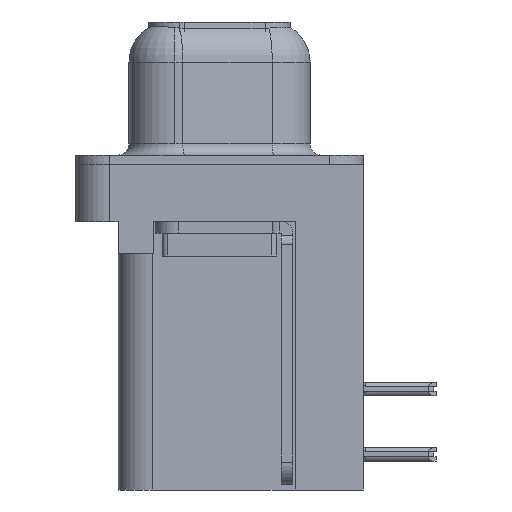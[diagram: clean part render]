
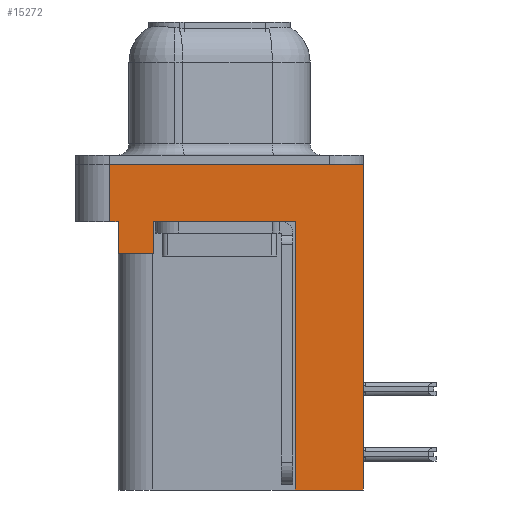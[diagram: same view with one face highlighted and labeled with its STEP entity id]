
A CAD part, left-side view. The second image highlights one B-rep face of the part: STEP entity #15272.
In plain terms, the highlighted planar face has unit normal (-1, 0, 0).
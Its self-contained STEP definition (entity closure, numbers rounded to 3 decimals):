
#4 = LINE ( 'NONE', #18601, #1381 ) ;
#1381 = VECTOR ( 'NONE', #23436, 1000. ) ;
#2305 = VERTEX_POINT ( 'NONE', #29131 ) ;
#3028 = EDGE_CURVE ( 'NONE', #26941, #27357, #26140, .T. ) ;
#3151 = EDGE_CURVE ( 'NONE', #13472, #6666, #7966, .T. ) ;
#3356 = LINE ( 'NONE', #11405, #26285 ) ;
#3766 = DIRECTION ( 'NONE',  ( 0., 0., 1. ) ) ;
#3957 = ORIENTED_EDGE ( 'NONE', *, *, #4038, .F. ) ;
#4038 = EDGE_CURVE ( 'NONE', #20231, #8632, #13422, .T. ) ;
#4247 = CARTESIAN_POINT ( 'NONE',  ( -3., 2.895, -3.9 ) ) ;
#4340 = VERTEX_POINT ( 'NONE', #17280 ) ;
#4363 = CARTESIAN_POINT ( 'NONE',  ( -3., 4.425, -3.9 ) ) ;
#4394 = EDGE_CURVE ( 'NONE', #6666, #2305, #20067, .T. ) ;
#4581 = DIRECTION ( 'NONE',  ( 0., 1., 0. ) ) ;
#4609 = CARTESIAN_POINT ( 'NONE',  ( -3., 4.425, -2.5 ) ) ;
#4730 = LINE ( 'NONE', #12021, #21700 ) ;
#4919 = VECTOR ( 'NONE', #22913, 1000. ) ;
#5632 = DIRECTION ( 'NONE',  ( 0., -1., 0. ) ) ;
#5681 = VECTOR ( 'NONE', #7447, 1000. ) ;
#5896 = CARTESIAN_POINT ( 'NONE',  ( -3., -6.275, -14.2 ) ) ;
#6021 = ORIENTED_EDGE ( 'NONE', *, *, #4394, .T. ) ;
#6219 = DIRECTION ( 'NONE',  ( 0., 1., 0. ) ) ;
#6666 = VERTEX_POINT ( 'NONE', #14466 ) ;
#7362 = DIRECTION ( 'NONE',  ( 0., 0., 1. ) ) ;
#7447 = DIRECTION ( 'NONE',  ( 0., 0., 1. ) ) ;
#7614 = PLANE ( 'NONE',  #14154 ) ;
#7671 = ORIENTED_EDGE ( 'NONE', *, *, #15102, .T. ) ;
#7966 = LINE ( 'NONE', #8420, #30158 ) ;
#8420 = CARTESIAN_POINT ( 'NONE',  ( -3., 2.895, -3.9 ) ) ;
#8632 = VERTEX_POINT ( 'NONE', #16535 ) ;
#8989 = CARTESIAN_POINT ( 'NONE',  ( -3., 4.425, -3.9 ) ) ;
#9892 = VECTOR ( 'NONE', #5632, 1000. ) ;
#10403 = VERTEX_POINT ( 'NONE', #5896 ) ;
#11405 = CARTESIAN_POINT ( 'NONE',  ( -3., -3.295, -14.2 ) ) ;
#12021 = CARTESIAN_POINT ( 'NONE',  ( -3., 4.775, -2.5 ) ) ;
#12225 = VECTOR ( 'NONE', #23926, 1000. ) ;
#12559 = CARTESIAN_POINT ( 'NONE',  ( -3., -6.275, -2.5 ) ) ;
#13422 = LINE ( 'NONE', #27539, #4919 ) ;
#13472 = VERTEX_POINT ( 'NONE', #4247 ) ;
#13940 = EDGE_CURVE ( 'NONE', #13472, #26941, #20506, .T. ) ;
#14154 = AXIS2_PLACEMENT_3D ( 'NONE', #12559, #17077, #26540 ) ;
#14466 = CARTESIAN_POINT ( 'NONE',  ( -3., 2.895, -2.5 ) ) ;
#14591 = CARTESIAN_POINT ( 'NONE',  ( -3., -6.275, -2.5 ) ) ;
#15102 = EDGE_CURVE ( 'NONE', #10403, #8632, #16470, .T. ) ;
#15272 = ADVANCED_FACE ( 'NONE', ( #24377 ), #7614, .T. ) ;
#15326 = ORIENTED_EDGE ( 'NONE', *, *, #3028, .F. ) ;
#16470 = LINE ( 'NONE', #14591, #12225 ) ;
#16535 = CARTESIAN_POINT ( 'NONE',  ( -3., -6.275, 0. ) ) ;
#17077 = DIRECTION ( 'NONE',  ( -1., 0., 0. ) ) ;
#17280 = CARTESIAN_POINT ( 'NONE',  ( -3., 4.775, -2.5 ) ) ;
#17578 = CARTESIAN_POINT ( 'NONE',  ( -3., -6.275, -2.5 ) ) ;
#18377 = EDGE_CURVE ( 'NONE', #22040, #2305, #21432, .T. ) ;
#18601 = CARTESIAN_POINT ( 'NONE',  ( -3., -6.275, -2.5 ) ) ;
#18868 = ORIENTED_EDGE ( 'NONE', *, *, #3151, .T. ) ;
#20067 = LINE ( 'NONE', #17578, #9892 ) ;
#20231 = VERTEX_POINT ( 'NONE', #22662 ) ;
#20240 = ORIENTED_EDGE ( 'NONE', *, *, #18377, .F. ) ;
#20506 = LINE ( 'NONE', #4363, #30233 ) ;
#21024 = CARTESIAN_POINT ( 'NONE',  ( -3., -3.295, -14.2 ) ) ;
#21432 = LINE ( 'NONE', #26836, #5681 ) ;
#21640 = ORIENTED_EDGE ( 'NONE', *, *, #13940, .F. ) ;
#21647 = CARTESIAN_POINT ( 'NONE',  ( -3., 4.425, -3.9 ) ) ;
#21700 = VECTOR ( 'NONE', #7362, 1000. ) ;
#21826 = ORIENTED_EDGE ( 'NONE', *, *, #26031, .T. ) ;
#22040 = VERTEX_POINT ( 'NONE', #21024 ) ;
#22248 = VECTOR ( 'NONE', #29052, 1000. ) ;
#22662 = CARTESIAN_POINT ( 'NONE',  ( -3., 4.775, 0. ) ) ;
#22913 = DIRECTION ( 'NONE',  ( 0., -1., 0. ) ) ;
#23139 = EDGE_CURVE ( 'NONE', #4340, #20231, #4730, .T. ) ;
#23436 = DIRECTION ( 'NONE',  ( 0., -1., 0. ) ) ;
#23926 = DIRECTION ( 'NONE',  ( 0., 0., 1. ) ) ;
#24377 = FACE_OUTER_BOUND ( 'NONE', #30581, .T. ) ;
#24516 = ORIENTED_EDGE ( 'NONE', *, *, #28962, .F. ) ;
#26031 = EDGE_CURVE ( 'NONE', #4340, #27357, #4, .T. ) ;
#26140 = LINE ( 'NONE', #21647, #22248 ) ;
#26285 = VECTOR ( 'NONE', #4581, 1000. ) ;
#26540 = DIRECTION ( 'NONE',  ( 0., 0., 1. ) ) ;
#26836 = CARTESIAN_POINT ( 'NONE',  ( -3., -3.295, -14.2 ) ) ;
#26941 = VERTEX_POINT ( 'NONE', #8989 ) ;
#27357 = VERTEX_POINT ( 'NONE', #4609 ) ;
#27539 = CARTESIAN_POINT ( 'NONE',  ( -3., -6.275, 0. ) ) ;
#28334 = ORIENTED_EDGE ( 'NONE', *, *, #23139, .F. ) ;
#28962 = EDGE_CURVE ( 'NONE', #10403, #22040, #3356, .T. ) ;
#29052 = DIRECTION ( 'NONE',  ( 0., 0., 1. ) ) ;
#29131 = CARTESIAN_POINT ( 'NONE',  ( -3., -3.295, -2.5 ) ) ;
#30158 = VECTOR ( 'NONE', #3766, 1000. ) ;
#30233 = VECTOR ( 'NONE', #6219, 1000. ) ;
#30581 = EDGE_LOOP ( 'NONE', ( #3957, #28334, #21826, #15326, #21640, #18868, #6021, #20240, #24516, #7671 ) ) ;
